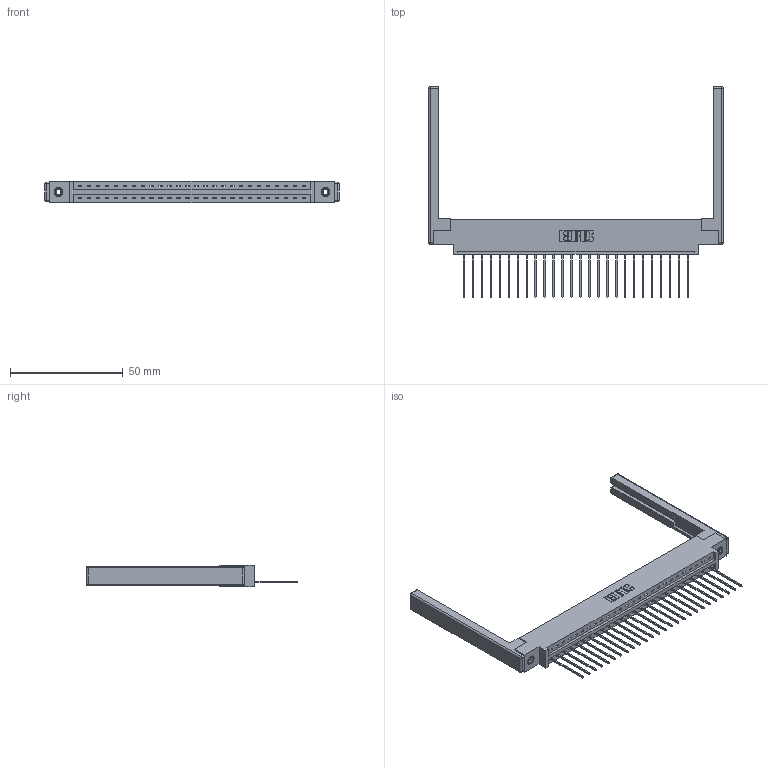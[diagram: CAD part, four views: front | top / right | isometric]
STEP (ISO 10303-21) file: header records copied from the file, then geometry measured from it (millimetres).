
FILE_DESCRIPTION (( 'STEP AP203' ), '1' );
FILE_NAME ('387-026-541-668.STEP', '2019-10-03T12:54:00', ( '' ), ( '' ), 'SwSTEP 2.0', 'SolidWorks 2016', '' );
FILE_SCHEMA (( 'CONFIG_CONTROL_DESIGN' ));
Length unit declared in the file: inch
Products named in the file (5): 337 Part_0.170 Offset - 0.156 Dia-TI; 307-220-068; 387-026-541-668; 345-250-001_345-250-001-102; 345-292-001_345-293-141
Assembly tree (31 placements, depth 2):
  387-026-541-668
    337 Part_0.170 Offset - 0.156 Dia-TI
    345-292-001_345-293-141  x26
    345-250-001_345-250-001-102  x2
    307-220-068  x2
Bounding box: 130.45 x 93.35 x 9.4 mm (x, y, z)
Volume: 17717.8 mm3; surface area: 18399.1 mm2
Topology: 31 solids, 31 shells, 1884 faces, 5601 edges, 3678 vertices
Faces by surface type: plane 1358, cylinder 502, cone 12, sphere 8, torus 4
Entity records: 24306 total; most frequent: CARTESIAN_POINT 4189, ORIENTED_EDGE 4140, DIRECTION 3632, EDGE_CURVE 2070, VECTOR 1892, LINE 1892, VERTEX_POINT 1370, AXIS2_PLACEMENT_3D 870
